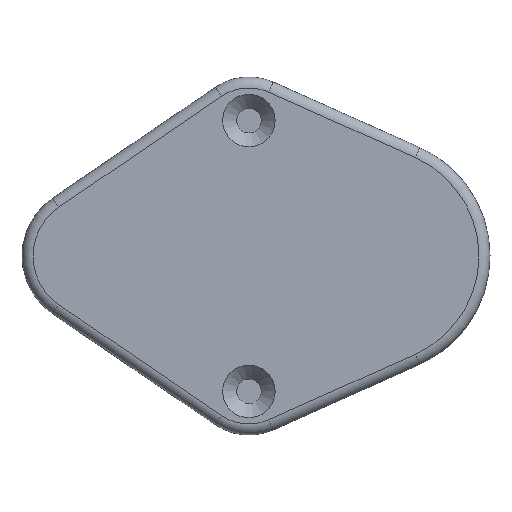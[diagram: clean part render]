
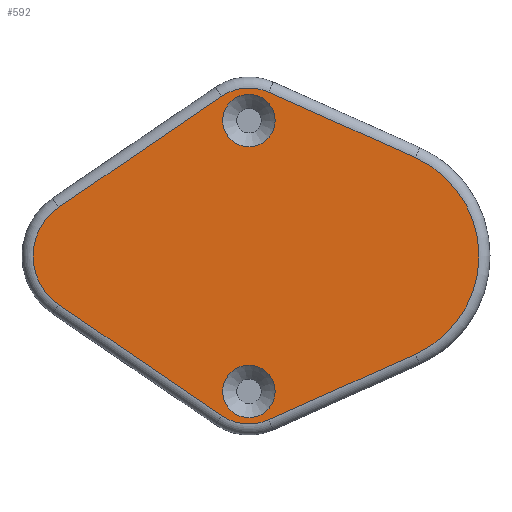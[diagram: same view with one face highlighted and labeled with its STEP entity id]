
A CAD part, top view. The second image highlights one B-rep face of the part: STEP entity #592.
In plain terms, the highlighted planar face has unit normal (0, 0, 1).
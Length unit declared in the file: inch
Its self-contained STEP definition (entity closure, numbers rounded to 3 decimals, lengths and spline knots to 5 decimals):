
#36 = CARTESIAN_POINT ( 'NONE',  ( 0.94376, 0.70411, 0.5 ) ) ;
#38 = CARTESIAN_POINT ( 'NONE',  ( -0.4416, 1.14311, 0.5 ) ) ;
#60 = CIRCLE ( 'NONE', #359, 0.34626 ) ;
#65 = EDGE_CURVE ( 'NONE', #602, #756, #1302, .T. ) ;
#68 = DIRECTION ( 'NONE',  ( 1., 0., 0. ) ) ;
#92 = DIRECTION ( 'NONE',  ( 1., 0., 0. ) ) ;
#95 = CARTESIAN_POINT ( 'NONE',  ( -1.371, 0., 0.5 ) ) ;
#116 = CARTESIAN_POINT ( 'NONE',  ( 0., 0., 0.5 ) ) ;
#117 = CARTESIAN_POINT ( 'NONE',  ( -0.4416, -1.14311, 0.5 ) ) ;
#145 = CIRCLE ( 'NONE', #1158, 0.34626 ) ;
#165 = DIRECTION ( 'NONE',  ( 1., 0., 0. ) ) ;
#192 = DIRECTION ( 'NONE',  ( -0.913, 0.408, 0. ) ) ;
#195 = EDGE_CURVE ( 'NONE', #739, #1050, #469, .T. ) ;
#198 = AXIS2_PLACEMENT_3D ( 'NONE', #1173, #609, #165 ) ;
#222 = DIRECTION ( 'NONE',  ( 0.913, 0.408, 0. ) ) ;
#224 = AXIS2_PLACEMENT_3D ( 'NONE', #1113, #459, #1226 ) ;
#226 = VECTOR ( 'NONE', #670, 39.37008 ) ;
#238 = LINE ( 'NONE', #1104, #226 ) ;
#251 = CIRCLE ( 'NONE', #958, 0.188 ) ;
#259 = EDGE_CURVE ( 'NONE', #756, #739, #450, .T. ) ;
#261 = CARTESIAN_POINT ( 'NONE',  ( -0.10529, 1.17308, 0.5 ) ) ;
#267 = CIRCLE ( 'NONE', #1289, 0.42126 ) ;
#287 = ORIENTED_EDGE ( 'NONE', *, *, #1252, .T. ) ;
#325 = FACE_BOUND ( 'NONE', #740, .T. ) ;
#327 = FACE_OUTER_BOUND ( 'NONE', #620, .T. ) ;
#349 = CARTESIAN_POINT ( 'NONE',  ( -0.05861, -0.96897, 0.5 ) ) ;
#359 = AXIS2_PLACEMENT_3D ( 'NONE', #401, #1161, #507 ) ;
#374 = FACE_BOUND ( 'NONE', #853, .T. ) ;
#401 = CARTESIAN_POINT ( 'NONE',  ( -0.24661, -0.85697, 0.5 ) ) ;
#422 = VECTOR ( 'NONE', #192, 39.37008 ) ;
#450 = CIRCLE ( 'NONE', #198, 0.77126 ) ;
#459 = DIRECTION ( 'NONE',  ( 0., 0., 1. ) ) ;
#469 = LINE ( 'NONE', #494, #422 ) ;
#474 = CARTESIAN_POINT ( 'NONE',  ( -0.24661, 0.85697, 0.5 ) ) ;
#476 = VECTOR ( 'NONE', #222, 39.37008 ) ;
#494 = CARTESIAN_POINT ( 'NONE',  ( -0.10529, 1.17308, 0.5 ) ) ;
#507 = DIRECTION ( 'NONE',  ( 1., 0., 0. ) ) ;
#513 = ORIENTED_EDGE ( 'NONE', *, *, #713, .T. ) ;
#547 = CARTESIAN_POINT ( 'NONE',  ( -0.24661, -0.96897, 0.5 ) ) ;
#548 = DIRECTION ( 'NONE',  ( 1., 0., 0. ) ) ;
#559 = DIRECTION ( 'NONE',  ( 0., 0., 1. ) ) ;
#560 = ORIENTED_EDGE ( 'NONE', *, *, #1401, .F. ) ;
#569 = DIRECTION ( 'NONE',  ( 1., 0., 0. ) ) ;
#577 = ORIENTED_EDGE ( 'NONE', *, *, #768, .T. ) ;
#592 = ADVANCED_FACE ( 'NONE', ( #327, #374, #325 ), #658, .T. ) ;
#602 = VERTEX_POINT ( 'NONE', #1268 ) ;
#609 = DIRECTION ( 'NONE',  ( 0., 0., 1. ) ) ;
#618 = AXIS2_PLACEMENT_3D ( 'NONE', #116, #559, #92 ) ;
#620 = EDGE_LOOP ( 'NONE', ( #1083, #1018, #1132, #694, #287, #513, #577, #649 ) ) ;
#649 = ORIENTED_EDGE ( 'NONE', *, *, #1140, .T. ) ;
#658 = PLANE ( 'NONE',  #618 ) ;
#670 = DIRECTION ( 'NONE',  ( 0.826, -0.563, 0. ) ) ;
#679 = CARTESIAN_POINT ( 'NONE',  ( -0.05861, 0.96897, 0.5 ) ) ;
#694 = ORIENTED_EDGE ( 'NONE', *, *, #1020, .T. ) ;
#713 = EDGE_CURVE ( 'NONE', #1099, #935, #267, .T. ) ;
#739 = VERTEX_POINT ( 'NONE', #36 ) ;
#740 = EDGE_LOOP ( 'NONE', ( #914 ) ) ;
#756 = VERTEX_POINT ( 'NONE', #989 ) ;
#759 = EDGE_CURVE ( 'NONE', #966, #966, #251, .T. ) ;
#764 = CARTESIAN_POINT ( 'NONE',  ( -1.60822, 0.34812, 0.5 ) ) ;
#768 = EDGE_CURVE ( 'NONE', #935, #962, #238, .T. ) ;
#779 = VERTEX_POINT ( 'NONE', #679 ) ;
#804 = VERTEX_POINT ( 'NONE', #38 ) ;
#853 = EDGE_LOOP ( 'NONE', ( #560 ) ) ;
#872 = DIRECTION ( 'NONE',  ( -0.826, -0.563, 0. ) ) ;
#914 = ORIENTED_EDGE ( 'NONE', *, *, #759, .F. ) ;
#935 = VERTEX_POINT ( 'NONE', #1187 ) ;
#958 = AXIS2_PLACEMENT_3D ( 'NONE', #547, #1337, #548 ) ;
#962 = VERTEX_POINT ( 'NONE', #117 ) ;
#966 = VERTEX_POINT ( 'NONE', #349 ) ;
#989 = CARTESIAN_POINT ( 'NONE',  ( 0.94376, -0.70411, 0.5 ) ) ;
#1018 = ORIENTED_EDGE ( 'NONE', *, *, #259, .T. ) ;
#1020 = EDGE_CURVE ( 'NONE', #1050, #804, #145, .T. ) ;
#1050 = VERTEX_POINT ( 'NONE', #261 ) ;
#1061 = DIRECTION ( 'NONE',  ( 0., 0., 1. ) ) ;
#1083 = ORIENTED_EDGE ( 'NONE', *, *, #65, .T. ) ;
#1099 = VERTEX_POINT ( 'NONE', #1258 ) ;
#1104 = CARTESIAN_POINT ( 'NONE',  ( -0.67198, -0.98611, 0.5 ) ) ;
#1113 = CARTESIAN_POINT ( 'NONE',  ( -0.24661, 0.96897, 0.5 ) ) ;
#1132 = ORIENTED_EDGE ( 'NONE', *, *, #195, .T. ) ;
#1140 = EDGE_CURVE ( 'NONE', #962, #602, #60, .T. ) ;
#1158 = AXIS2_PLACEMENT_3D ( 'NONE', #474, #1241, #569 ) ;
#1161 = DIRECTION ( 'NONE',  ( 0., 0., 1. ) ) ;
#1173 = CARTESIAN_POINT ( 'NONE',  ( 0.629, 0., 0.5 ) ) ;
#1187 = CARTESIAN_POINT ( 'NONE',  ( -1.60822, -0.34812, 0.5 ) ) ;
#1226 = DIRECTION ( 'NONE',  ( 1., 0., 0. ) ) ;
#1241 = DIRECTION ( 'NONE',  ( 0., 0., 1. ) ) ;
#1252 = EDGE_CURVE ( 'NONE', #804, #1099, #1396, .T. ) ;
#1258 = CARTESIAN_POINT ( 'NONE',  ( -1.60822, 0.34812, 0.5 ) ) ;
#1268 = CARTESIAN_POINT ( 'NONE',  ( -0.10529, -1.17308, 0.5 ) ) ;
#1289 = AXIS2_PLACEMENT_3D ( 'NONE', #95, #1061, #68 ) ;
#1298 = CARTESIAN_POINT ( 'NONE',  ( 0.41953, -0.93846, 0.5 ) ) ;
#1302 = LINE ( 'NONE', #1298, #476 ) ;
#1337 = DIRECTION ( 'NONE',  ( 0., 0., 1. ) ) ;
#1378 = CIRCLE ( 'NONE', #224, 0.188 ) ;
#1394 = VECTOR ( 'NONE', #872, 39.37008 ) ;
#1396 = LINE ( 'NONE', #764, #1394 ) ;
#1401 = EDGE_CURVE ( 'NONE', #779, #779, #1378, .T. ) ;
